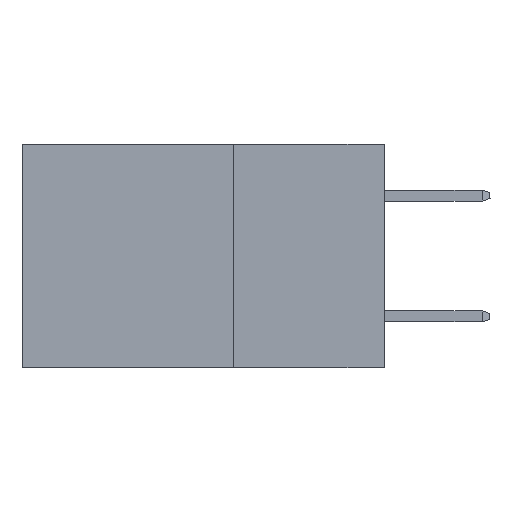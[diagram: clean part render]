
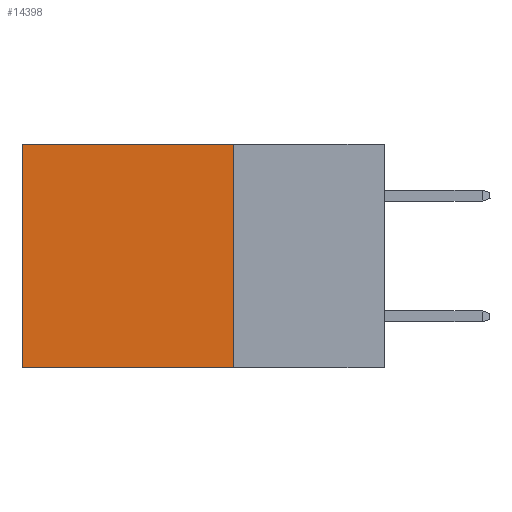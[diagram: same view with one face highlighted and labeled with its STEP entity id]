
A CAD part, left-side view. The second image highlights one B-rep face of the part: STEP entity #14398.
In plain terms, the highlighted planar face has unit normal (-1, 0, 0).
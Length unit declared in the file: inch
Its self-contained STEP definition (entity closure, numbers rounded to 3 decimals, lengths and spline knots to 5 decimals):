
#1126 = CARTESIAN_POINT ( 'NONE',  ( 0.298, 0.6, -0.37 ) ) ;
#1507 = EDGE_LOOP ( 'NONE', ( #20938, #3914, #22620, #25350 ) ) ;
#2964 = CARTESIAN_POINT ( 'NONE',  ( 0.298, 0.25, 0. ) ) ;
#3914 = ORIENTED_EDGE ( 'NONE', *, *, #5038, .F. ) ;
#4639 = VERTEX_POINT ( 'NONE', #21507 ) ;
#4929 = CARTESIAN_POINT ( 'NONE',  ( 0.298, 0.6, 0. ) ) ;
#5038 = EDGE_CURVE ( 'NONE', #21491, #17336, #24290, .T. ) ;
#5411 = VECTOR ( 'NONE', #19808, 39.37008 ) ;
#7748 = LINE ( 'NONE', #2964, #23985 ) ;
#9305 = PLANE ( 'NONE',  #15363 ) ;
#9311 = DIRECTION ( 'NONE',  ( 0., 0., -1. ) ) ;
#10969 = CARTESIAN_POINT ( 'NONE',  ( 0.298, 0.25, 0. ) ) ;
#11431 = DIRECTION ( 'NONE',  ( 0., 0., -1. ) ) ;
#11703 = EDGE_CURVE ( 'NONE', #4639, #21491, #7748, .T. ) ;
#14398 = ADVANCED_FACE ( 'NONE', ( #23546 ), #9305, .F. ) ;
#15363 = AXIS2_PLACEMENT_3D ( 'NONE', #15641, #24142, #11431 ) ;
#15636 = VERTEX_POINT ( 'NONE', #21879 ) ;
#15641 = CARTESIAN_POINT ( 'NONE',  ( 0.298, 0.25, 0. ) ) ;
#16046 = LINE ( 'NONE', #4929, #5411 ) ;
#16718 = CARTESIAN_POINT ( 'NONE',  ( 0.298, 0.25, -0.37 ) ) ;
#17336 = VERTEX_POINT ( 'NONE', #1126 ) ;
#18344 = VECTOR ( 'NONE', #25785, 39.37008 ) ;
#19808 = DIRECTION ( 'NONE',  ( 0., 0., -1. ) ) ;
#20525 = EDGE_CURVE ( 'NONE', #15636, #17336, #16046, .T. ) ;
#20938 = ORIENTED_EDGE ( 'NONE', *, *, #20525, .T. ) ;
#21491 = VERTEX_POINT ( 'NONE', #16718 ) ;
#21507 = CARTESIAN_POINT ( 'NONE',  ( 0.298, 0.25, 0. ) ) ;
#21879 = CARTESIAN_POINT ( 'NONE',  ( 0.298, 0.6, 0. ) ) ;
#22620 = ORIENTED_EDGE ( 'NONE', *, *, #11703, .F. ) ;
#23160 = EDGE_CURVE ( 'NONE', #4639, #15636, #23941, .T. ) ;
#23546 = FACE_OUTER_BOUND ( 'NONE', #1507, .T. ) ;
#23639 = VECTOR ( 'NONE', #26331, 39.37008 ) ;
#23941 = LINE ( 'NONE', #10969, #18344 ) ;
#23985 = VECTOR ( 'NONE', #9311, 39.37008 ) ;
#24142 = DIRECTION ( 'NONE',  ( 1., 0., 0. ) ) ;
#24263 = CARTESIAN_POINT ( 'NONE',  ( 0.298, 0.25, -0.37 ) ) ;
#24290 = LINE ( 'NONE', #24263, #23639 ) ;
#25350 = ORIENTED_EDGE ( 'NONE', *, *, #23160, .T. ) ;
#25785 = DIRECTION ( 'NONE',  ( 0., 1., 0. ) ) ;
#26331 = DIRECTION ( 'NONE',  ( 0., 1., 0. ) ) ;
